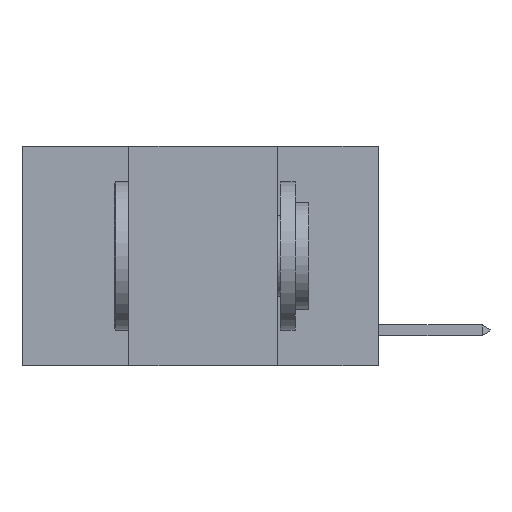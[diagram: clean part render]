
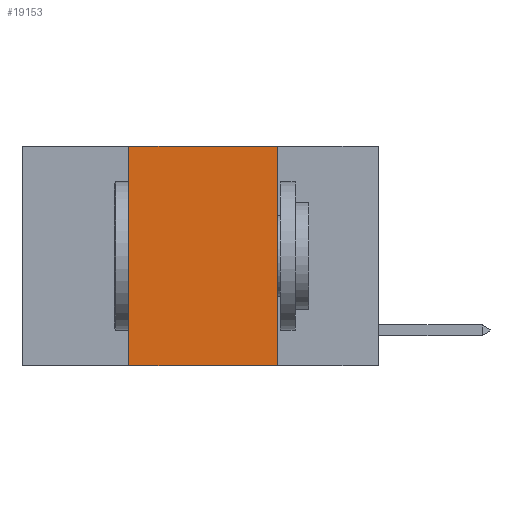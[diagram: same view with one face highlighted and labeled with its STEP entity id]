
A CAD part, left-side view. The second image highlights one B-rep face of the part: STEP entity #19153.
In plain terms, the highlighted planar face has unit normal (-1, 0, 0).
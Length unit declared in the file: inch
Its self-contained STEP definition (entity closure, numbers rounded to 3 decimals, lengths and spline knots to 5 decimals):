
#64 = DIRECTION ( 'NONE',  ( 0., -1., 0. ) ) ;
#134 = EDGE_CURVE ( 'NONE', #8742, #14816, #11443, .T. ) ;
#241 = ORIENTED_EDGE ( 'NONE', *, *, #3368, .T. ) ;
#2147 = PLANE ( 'NONE',  #21007 ) ;
#2893 = VECTOR ( 'NONE', #64, 39.37008 ) ;
#3368 = EDGE_CURVE ( 'NONE', #8742, #21277, #8100, .T. ) ;
#3408 = LINE ( 'NONE', #5522, #12169 ) ;
#3959 = CARTESIAN_POINT ( 'NONE',  ( 0., 0.6, 0. ) ) ;
#5522 = CARTESIAN_POINT ( 'NONE',  ( 0., 0.17, 0. ) ) ;
#5697 = CARTESIAN_POINT ( 'NONE',  ( 0., 0.6, 0. ) ) ;
#7422 = DIRECTION ( 'NONE',  ( 0., 0., -1. ) ) ;
#8100 = LINE ( 'NONE', #13995, #2893 ) ;
#8336 = DIRECTION ( 'NONE',  ( 0., 0., 1. ) ) ;
#8673 = ORIENTED_EDGE ( 'NONE', *, *, #22192, .F. ) ;
#8718 = LINE ( 'NONE', #3959, #22041 ) ;
#8742 = VERTEX_POINT ( 'NONE', #12401 ) ;
#9411 = EDGE_CURVE ( 'NONE', #19068, #21277, #3408, .T. ) ;
#11167 = FACE_OUTER_BOUND ( 'NONE', #14767, .T. ) ;
#11443 = LINE ( 'NONE', #18965, #20674 ) ;
#12169 = VECTOR ( 'NONE', #15935, 39.37008 ) ;
#12401 = CARTESIAN_POINT ( 'NONE',  ( 0., 0.42, -0.37 ) ) ;
#12596 = ORIENTED_EDGE ( 'NONE', *, *, #9411, .F. ) ;
#13769 = CARTESIAN_POINT ( 'NONE',  ( 0., 0.17, -0.37 ) ) ;
#13995 = CARTESIAN_POINT ( 'NONE',  ( 0., 0.6, -0.37 ) ) ;
#14767 = EDGE_LOOP ( 'NONE', ( #12596, #8673, #21744, #241 ) ) ;
#14816 = VERTEX_POINT ( 'NONE', #21908 ) ;
#15935 = DIRECTION ( 'NONE',  ( 0., 0., -1. ) ) ;
#16211 = DIRECTION ( 'NONE',  ( 0., -1., 0. ) ) ;
#17828 = DIRECTION ( 'NONE',  ( 1., 0., 0. ) ) ;
#18965 = CARTESIAN_POINT ( 'NONE',  ( 0., 0.42, 0. ) ) ;
#19068 = VERTEX_POINT ( 'NONE', #19366 ) ;
#19153 = ADVANCED_FACE ( 'NONE', ( #11167 ), #2147, .F. ) ;
#19366 = CARTESIAN_POINT ( 'NONE',  ( 0., 0.17, 0. ) ) ;
#20674 = VECTOR ( 'NONE', #8336, 39.37008 ) ;
#21007 = AXIS2_PLACEMENT_3D ( 'NONE', #5697, #17828, #7422 ) ;
#21277 = VERTEX_POINT ( 'NONE', #13769 ) ;
#21744 = ORIENTED_EDGE ( 'NONE', *, *, #134, .F. ) ;
#21908 = CARTESIAN_POINT ( 'NONE',  ( 0., 0.42, 0. ) ) ;
#22041 = VECTOR ( 'NONE', #16211, 39.37008 ) ;
#22192 = EDGE_CURVE ( 'NONE', #14816, #19068, #8718, .T. ) ;
